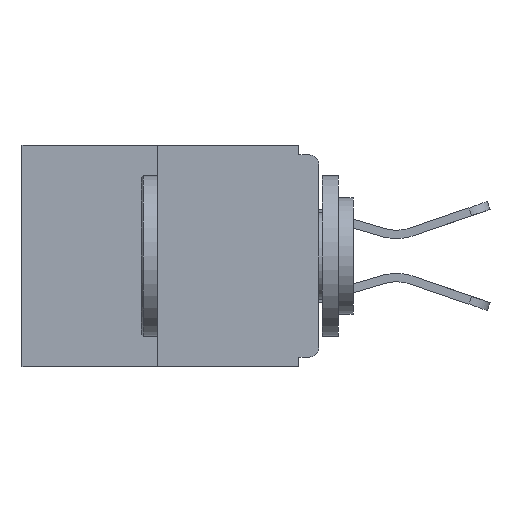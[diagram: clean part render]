
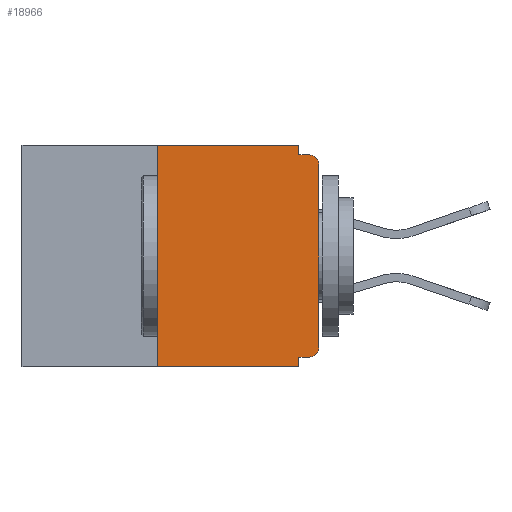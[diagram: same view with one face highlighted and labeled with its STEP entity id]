
A CAD part, left-side view. The second image highlights one B-rep face of the part: STEP entity #18966.
In plain terms, the highlighted planar face has unit normal (-1, 0, 0).
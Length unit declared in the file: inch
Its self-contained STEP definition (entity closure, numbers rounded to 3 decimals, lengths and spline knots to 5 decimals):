
#189 = EDGE_CURVE ( 'NONE', #3131, #17977, #11515, .T. ) ;
#322 = VERTEX_POINT ( 'NONE', #24002 ) ;
#517 = VERTEX_POINT ( 'NONE', #22738 ) ;
#696 = EDGE_CURVE ( 'NONE', #24831, #12600, #19019, .T. ) ;
#1171 = VECTOR ( 'NONE', #12132, 39.37008 ) ;
#1614 = CARTESIAN_POINT ( 'NONE',  ( 0., 0.031, 0. ) ) ;
#1686 = DIRECTION ( 'NONE',  ( 0., 0., -1. ) ) ;
#1775 = ORIENTED_EDGE ( 'NONE', *, *, #1803, .F. ) ;
#1803 = EDGE_CURVE ( 'NONE', #517, #7640, #14464, .T. ) ;
#2124 = AXIS2_PLACEMENT_3D ( 'NONE', #17404, #7802, #1686 ) ;
#2255 = CARTESIAN_POINT ( 'NONE',  ( 0., 0.25, 0. ) ) ;
#3042 = DIRECTION ( 'NONE',  ( 0., 0., -1. ) ) ;
#3131 = VERTEX_POINT ( 'NONE', #19733 ) ;
#3317 = EDGE_CURVE ( 'NONE', #322, #24831, #11095, .T. ) ;
#3338 = CIRCLE ( 'NONE', #2124, 0.015 ) ;
#3763 = VECTOR ( 'NONE', #14448, 39.37008 ) ;
#3814 = AXIS2_PLACEMENT_3D ( 'NONE', #10557, #4904, #3042 ) ;
#3963 = VECTOR ( 'NONE', #7785, 39.37008 ) ;
#4191 = VECTOR ( 'NONE', #12828, 39.37008 ) ;
#4362 = DIRECTION ( 'NONE',  ( -1., 0., 0. ) ) ;
#4469 = ORIENTED_EDGE ( 'NONE', *, *, #189, .F. ) ;
#4532 = CARTESIAN_POINT ( 'NONE',  ( 0., 0.031, -0.343 ) ) ;
#4904 = DIRECTION ( 'NONE',  ( 1., 0., 0. ) ) ;
#5301 = CARTESIAN_POINT ( 'NONE',  ( 0., 0., 0. ) ) ;
#5364 = EDGE_CURVE ( 'NONE', #7640, #6874, #14060, .T. ) ;
#6127 = DIRECTION ( 'NONE',  ( 0., -1., 0. ) ) ;
#6750 = LINE ( 'NONE', #1614, #12796 ) ;
#6824 = VECTOR ( 'NONE', #22865, 39.37008 ) ;
#6874 = VERTEX_POINT ( 'NONE', #13452 ) ;
#7244 = DIRECTION ( 'NONE',  ( 0., 0., 1. ) ) ;
#7310 = LINE ( 'NONE', #5301, #15522 ) ;
#7640 = VERTEX_POINT ( 'NONE', #2255 ) ;
#7682 = CARTESIAN_POINT ( 'NONE',  ( 0., 0.015, -0.015 ) ) ;
#7785 = DIRECTION ( 'NONE',  ( 0., -1., 0. ) ) ;
#7802 = DIRECTION ( 'NONE',  ( -1., 0., 0. ) ) ;
#8365 = ORIENTED_EDGE ( 'NONE', *, *, #15056, .T. ) ;
#9145 = DIRECTION ( 'NONE',  ( 0., 0., -1. ) ) ;
#10389 = ORIENTED_EDGE ( 'NONE', *, *, #5364, .F. ) ;
#10557 = CARTESIAN_POINT ( 'NONE',  ( 0., 0.46, 0. ) ) ;
#11027 = ORIENTED_EDGE ( 'NONE', *, *, #24569, .T. ) ;
#11095 = LINE ( 'NONE', #15198, #6824 ) ;
#11207 = VECTOR ( 'NONE', #6127, 39.37008 ) ;
#11515 = LINE ( 'NONE', #21764, #11207 ) ;
#12053 = EDGE_CURVE ( 'NONE', #24151, #17977, #14981, .T. ) ;
#12132 = DIRECTION ( 'NONE',  ( 0., 0., -1. ) ) ;
#12600 = VERTEX_POINT ( 'NONE', #18027 ) ;
#12796 = VECTOR ( 'NONE', #9145, 39.37008 ) ;
#12828 = DIRECTION ( 'NONE',  ( 0., 0., 1. ) ) ;
#13168 = CARTESIAN_POINT ( 'NONE',  ( 0., 0., -0.313 ) ) ;
#13170 = CARTESIAN_POINT ( 'NONE',  ( 0., 0.25, 0. ) ) ;
#13452 = CARTESIAN_POINT ( 'NONE',  ( 0., 0.031, 0. ) ) ;
#14060 = LINE ( 'NONE', #15250, #3763 ) ;
#14062 = ORIENTED_EDGE ( 'NONE', *, *, #3317, .F. ) ;
#14257 = DIRECTION ( 'NONE',  ( 0., 0., -1. ) ) ;
#14448 = DIRECTION ( 'NONE',  ( 0., -1., 0. ) ) ;
#14464 = LINE ( 'NONE', #13170, #4191 ) ;
#14925 = VERTEX_POINT ( 'NONE', #13168 ) ;
#14981 = CIRCLE ( 'NONE', #22579, 0.015 ) ;
#15056 = EDGE_CURVE ( 'NONE', #517, #12600, #20223, .T. ) ;
#15198 = CARTESIAN_POINT ( 'NONE',  ( 0., 0., -0.328 ) ) ;
#15250 = CARTESIAN_POINT ( 'NONE',  ( 0., 0.46, 0. ) ) ;
#15522 = VECTOR ( 'NONE', #7244, 39.37008 ) ;
#15809 = ORIENTED_EDGE ( 'NONE', *, *, #20130, .T. ) ;
#16246 = CARTESIAN_POINT ( 'NONE',  ( 0., 0., -0.03 ) ) ;
#17093 = ORIENTED_EDGE ( 'NONE', *, *, #12053, .T. ) ;
#17404 = CARTESIAN_POINT ( 'NONE',  ( 0., 0.015, -0.313 ) ) ;
#17482 = CARTESIAN_POINT ( 'NONE',  ( 0., 0.46, -0.343 ) ) ;
#17977 = VERTEX_POINT ( 'NONE', #7682 ) ;
#18027 = CARTESIAN_POINT ( 'NONE',  ( 0., 0.031, -0.343 ) ) ;
#18634 = PLANE ( 'NONE',  #3814 ) ;
#18750 = EDGE_LOOP ( 'NONE', ( #10389, #1775, #8365, #24273, #14062, #11027, #15809, #17093, #4469, #23034 ) ) ;
#18848 = CARTESIAN_POINT ( 'NONE',  ( 0., 0.031, -0.328 ) ) ;
#18966 = ADVANCED_FACE ( 'NONE', ( #24285 ), #18634, .F. ) ;
#19019 = LINE ( 'NONE', #4532, #1171 ) ;
#19140 = EDGE_CURVE ( 'NONE', #6874, #3131, #6750, .T. ) ;
#19733 = CARTESIAN_POINT ( 'NONE',  ( 0., 0.031, -0.015 ) ) ;
#20130 = EDGE_CURVE ( 'NONE', #14925, #24151, #7310, .T. ) ;
#20223 = LINE ( 'NONE', #17482, #3963 ) ;
#21587 = CARTESIAN_POINT ( 'NONE',  ( 0., 0.015, -0.03 ) ) ;
#21764 = CARTESIAN_POINT ( 'NONE',  ( 0., 0., -0.015 ) ) ;
#22579 = AXIS2_PLACEMENT_3D ( 'NONE', #21587, #4362, #14257 ) ;
#22738 = CARTESIAN_POINT ( 'NONE',  ( 0., 0.25, -0.343 ) ) ;
#22865 = DIRECTION ( 'NONE',  ( 0., 1., 0. ) ) ;
#23034 = ORIENTED_EDGE ( 'NONE', *, *, #19140, .F. ) ;
#24002 = CARTESIAN_POINT ( 'NONE',  ( 0., 0.015, -0.328 ) ) ;
#24151 = VERTEX_POINT ( 'NONE', #16246 ) ;
#24273 = ORIENTED_EDGE ( 'NONE', *, *, #696, .F. ) ;
#24285 = FACE_OUTER_BOUND ( 'NONE', #18750, .T. ) ;
#24569 = EDGE_CURVE ( 'NONE', #322, #14925, #3338, .T. ) ;
#24831 = VERTEX_POINT ( 'NONE', #18848 ) ;
